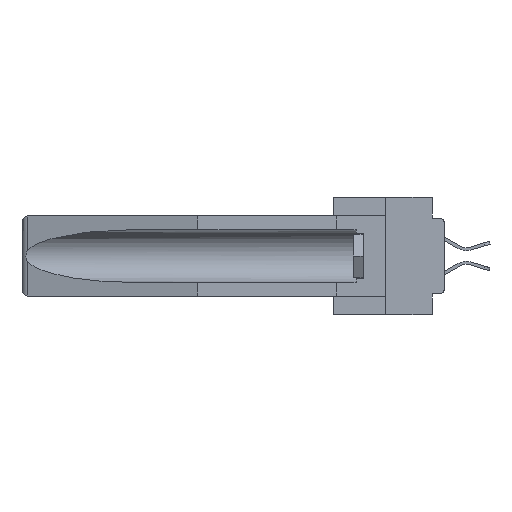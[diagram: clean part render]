
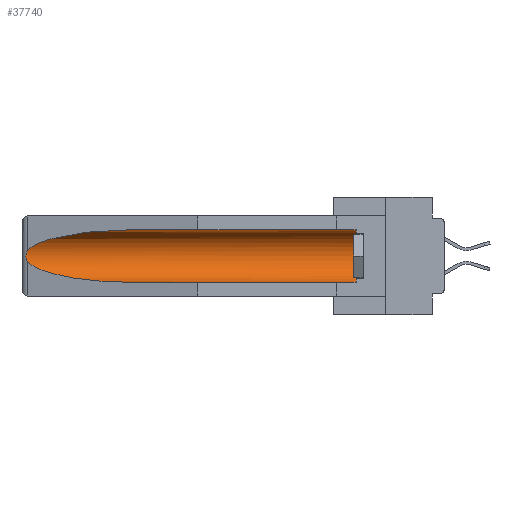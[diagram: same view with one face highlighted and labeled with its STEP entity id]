
A CAD part, left-side view. The second image highlights one B-rep face of the part: STEP entity #37740.
In plain terms, the highlighted cylindrical face has radius 2.857 mm (diameter 5.715 mm), a partial arc.
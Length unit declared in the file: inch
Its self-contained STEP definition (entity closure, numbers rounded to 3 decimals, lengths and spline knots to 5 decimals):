
#9 = VERTEX_POINT ( 'NONE', #4717 ) ;
#406 = CARTESIAN_POINT ( 'NONE',  ( 0.155, 0.126, -0.059 ) ) ;
#424 = VERTEX_POINT ( 'NONE', #12449 ) ;
#3747 = VERTEX_POINT ( 'NONE', #406 ) ;
#4405 = CARTESIAN_POINT ( 'NONE',  ( 0.2673, 1.53269, -0.17917 ) ) ;
#4614 = CARTESIAN_POINT ( 'NONE',  ( 0.155, -0.30754, -0.059 ) ) ;
#4717 = CARTESIAN_POINT ( 'NONE',  ( 0.155, 1.07973, -0.284 ) ) ;
#5537 = CARTESIAN_POINT ( 'NONE',  ( 0.155, -0.30754, -0.284 ) ) ;
#6241 = CARTESIAN_POINT ( 'NONE',  ( 0.155, -0.30754, -0.1715 ) ) ;
#6251 = EDGE_CURVE ( 'NONE', #12101, #26464, #19165, .T. ) ;
#6398 = FACE_OUTER_BOUND ( 'NONE', #31454, .T. ) ;
#6740 = CARTESIAN_POINT ( 'NONE',  ( 0.2675, 1.53308, -0.17534 ) ) ;
#6776 = EDGE_CURVE ( 'NONE', #3747, #12101, #35886, .T. ) ;
#6832 = CYLINDRICAL_SURFACE ( 'NONE', #21556, 0.1125 ) ;
#7693 = CARTESIAN_POINT ( 'NONE',  ( 0.21114, 1.30732, -0.284 ) ) ;
#8308 = CARTESIAN_POINT ( 'NONE',  ( 0.155, 0.126, -0.284 ) ) ;
#8466 = CARTESIAN_POINT ( 'NONE',  ( 0.155, 1.07973, -0.059 ) ) ;
#9559 = ORIENTED_EDGE ( 'NONE', *, *, #6776, .T. ) ;
#9658 = LINE ( 'NONE', #5537, #18677 ) ;
#9770 = CARTESIAN_POINT ( 'NONE',  ( 0.26655, 1.53094, -0.18657 ) ) ;
#10949 = CARTESIAN_POINT ( 'NONE',  ( 0.155, 1.07973, -0.284 ) ) ;
#12101 = VERTEX_POINT ( 'NONE', #8466 ) ;
#12449 = CARTESIAN_POINT ( 'NONE',  ( 0.26537, 1.52718, -0.19328 ) ) ;
#12583 = ORIENTED_EDGE ( 'NONE', *, *, #32771, .F. ) ;
#13057 = CARTESIAN_POINT ( 'NONE',  ( 0.26597, 1.52961, -0.15275 ) ) ;
#13389 = CARTESIAN_POINT ( 'NONE',  ( 0.26597, 1.5296, -0.19026 ) ) ;
#15238 = DIRECTION ( 'NONE',  ( 0., 1., 0. ) ) ;
#15738 = CARTESIAN_POINT ( 'NONE',  ( 0.26537, 1.52718, -0.14972 ) ) ;
#16118 = CARTESIAN_POINT ( 'NONE',  ( 0.2675, 1.53308, -0.16763 ) ) ;
#16346 = CARTESIAN_POINT ( 'NONE',  ( 0.21114, 1.30732, -0.059 ) ) ;
#17265 = EDGE_CURVE ( 'NONE', #26464, #424, #36868, .T. ) ;
#18677 = VECTOR ( 'NONE', #20979, 39.37008 ) ;
#19165 =( BOUNDED_CURVE ( )  B_SPLINE_CURVE ( 3, ( #26307, #16346, #35330, #37560 ),
 .UNSPECIFIED., .F., .F. ) 
 B_SPLINE_CURVE_WITH_KNOTS ( ( 4, 4 ),
 ( 4.71239, 6.08839 ),
 .UNSPECIFIED. ) 
 CURVE ( )  GEOMETRIC_REPRESENTATION_ITEM ( )  RATIONAL_B_SPLINE_CURVE ( ( 1., 0.848, 0.848, 1. ) ) 
 REPRESENTATION_ITEM ( '' )  );
#20979 = DIRECTION ( 'NONE',  ( 0., 1., 0. ) ) ;
#21004 = CARTESIAN_POINT ( 'NONE',  ( 0.26537, 1.52718, -0.14972 ) ) ;
#21556 = AXIS2_PLACEMENT_3D ( 'NONE', #6241, #15238, #27389 ) ;
#22350 = ORIENTED_EDGE ( 'NONE', *, *, #37360, .T. ) ;
#22843 =( BOUNDED_CURVE ( )  B_SPLINE_CURVE ( 3, ( #37164, #31205, #7693, #10949 ),
 .UNSPECIFIED., .F., .F. ) 
 B_SPLINE_CURVE_WITH_KNOTS ( ( 4, 4 ),
 ( 0.1948, 1.5708 ),
 .UNSPECIFIED. ) 
 CURVE ( )  GEOMETRIC_REPRESENTATION_ITEM ( )  RATIONAL_B_SPLINE_CURVE ( ( 1., 0.848, 0.848, 1. ) ) 
 REPRESENTATION_ITEM ( '' )  );
#23753 = DIRECTION ( 'NONE',  ( 0., 0., 1. ) ) ;
#24726 = ORIENTED_EDGE ( 'NONE', *, *, #6251, .T. ) ;
#24854 = CARTESIAN_POINT ( 'NONE',  ( 0.2673, 1.5327, -0.16383 ) ) ;
#26114 = CARTESIAN_POINT ( 'NONE',  ( 0.26537, 1.52718, -0.19328 ) ) ;
#26307 = CARTESIAN_POINT ( 'NONE',  ( 0.155, 1.07973, -0.059 ) ) ;
#26348 = VERTEX_POINT ( 'NONE', #8308 ) ;
#26464 = VERTEX_POINT ( 'NONE', #21004 ) ;
#27332 = ORIENTED_EDGE ( 'NONE', *, *, #33771, .T. ) ;
#27351 = ORIENTED_EDGE ( 'NONE', *, *, #17265, .T. ) ;
#27389 = DIRECTION ( 'NONE',  ( 0., 0., 1. ) ) ;
#27778 = VECTOR ( 'NONE', #28641, 39.37008 ) ;
#28641 = DIRECTION ( 'NONE',  ( 0., 1., 0. ) ) ;
#30994 = CIRCLE ( 'NONE', #32503, 0.1125 ) ;
#31205 = CARTESIAN_POINT ( 'NONE',  ( 0.25451, 1.48313, -0.24835 ) ) ;
#31454 = EDGE_LOOP ( 'NONE', ( #24726, #27351, #27332, #12583, #22350, #9559 ) ) ;
#32503 = AXIS2_PLACEMENT_3D ( 'NONE', #35540, #35803, #23753 ) ;
#32771 = EDGE_CURVE ( 'NONE', #26348, #9, #9658, .T. ) ;
#33771 = EDGE_CURVE ( 'NONE', #424, #9, #22843, .T. ) ;
#35330 = CARTESIAN_POINT ( 'NONE',  ( 0.25451, 1.48313, -0.09465 ) ) ;
#35540 = CARTESIAN_POINT ( 'NONE',  ( 0.155, 0.126, -0.1715 ) ) ;
#35803 = DIRECTION ( 'NONE',  ( 0., -1., 0. ) ) ;
#35886 = LINE ( 'NONE', #4614, #27778 ) ;
#36868 = B_SPLINE_CURVE_WITH_KNOTS ( 'NONE', 3,
 ( #15738, #13057, #36892, #24854, #16118, #6740, #4405, #9770, #13389, #26114 ),
 .UNSPECIFIED., .F., .F.,
 ( 4, 2, 2, 2, 4 ),
 ( 0., 0.00029, 0.00058, 0.00087, 0.00117 ),
 .UNSPECIFIED. ) ;
#36892 = CARTESIAN_POINT ( 'NONE',  ( 0.26654, 1.53092, -0.15636 ) ) ;
#37164 = CARTESIAN_POINT ( 'NONE',  ( 0.26537, 1.52718, -0.19328 ) ) ;
#37360 = EDGE_CURVE ( 'NONE', #26348, #3747, #30994, .T. ) ;
#37560 = CARTESIAN_POINT ( 'NONE',  ( 0.26537, 1.52718, -0.14972 ) ) ;
#37740 = ADVANCED_FACE ( 'NONE', ( #6398 ), #6832, .F. ) ;
